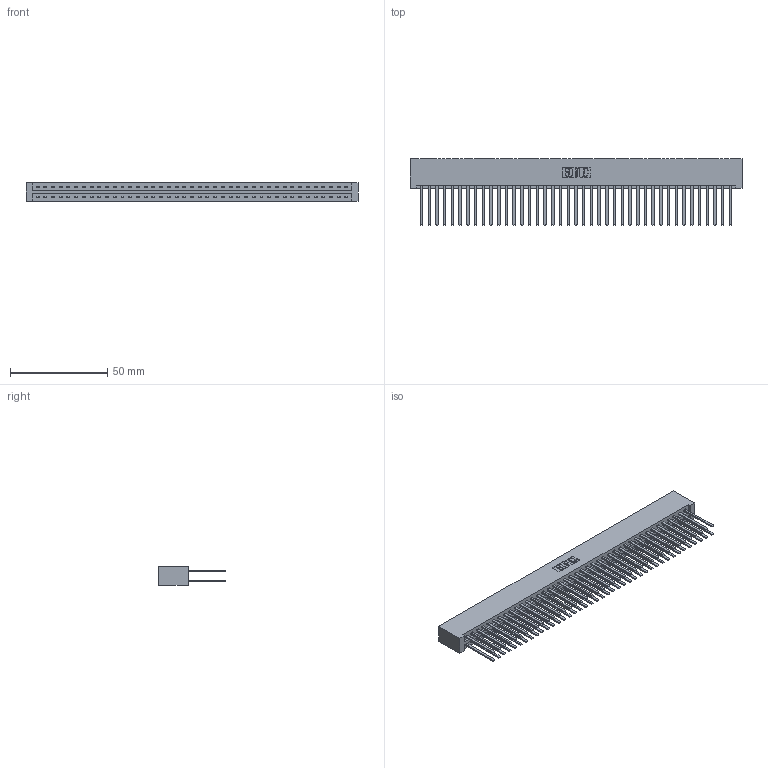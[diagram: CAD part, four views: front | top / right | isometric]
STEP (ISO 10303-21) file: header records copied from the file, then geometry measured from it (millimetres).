
FILE_DESCRIPTION (( 'STEP AP203' ), '1' );
FILE_NAME ('337-082-544-201.STEP', '2018-08-12T20:36:49', ( '' ), ( '' ), 'SwSTEP 2.0', 'SolidWorks 2016', '' );
FILE_SCHEMA (( 'CONFIG_CONTROL_DESIGN' ));
Length unit declared in the file: inch
Products named in the file (3): 337 Part_No Mounting Lugs; 345-292-001_345-293-144; 337-082-544-201
Assembly tree (83 placements, depth 2):
  337-082-544-201
    337 Part_No Mounting Lugs
    345-292-001_345-293-144  x82
Bounding box: 170.33 x 34.3 x 9.4 mm (x, y, z)
Volume: 19847.9 mm3; surface area: 26239.5 mm2
Topology: 83 solids, 83 shells, 4042 faces, 12013 edges, 7898 vertices
Faces by surface type: plane 2854, cylinder 1188
Entity records: 31457 total; most frequent: CARTESIAN_POINT 5298, ORIENTED_EDGE 5234, DIRECTION 4497, EDGE_CURVE 2617, LINE 2501, VECTOR 2501, VERTEX_POINT 1742, AXIS2_PLACEMENT_3D 998
